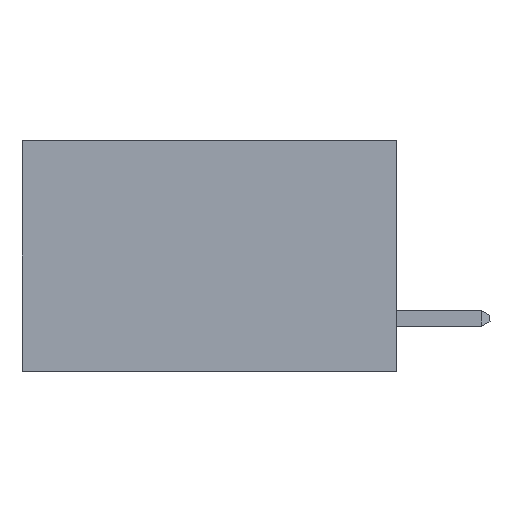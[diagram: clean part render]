
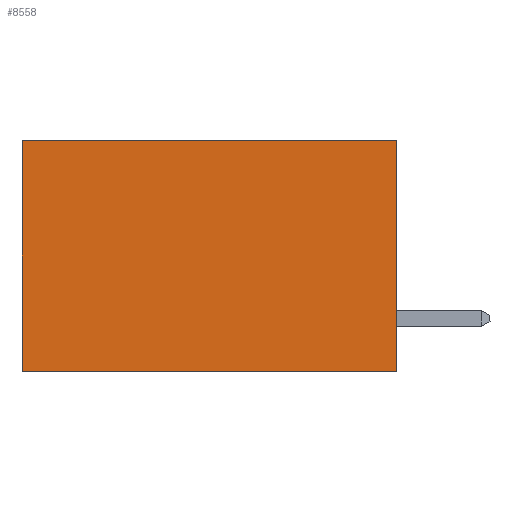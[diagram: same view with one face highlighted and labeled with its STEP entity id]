
A CAD part, left-side view. The second image highlights one B-rep face of the part: STEP entity #8558.
In plain terms, the highlighted planar face has unit normal (-1, 0, 0).
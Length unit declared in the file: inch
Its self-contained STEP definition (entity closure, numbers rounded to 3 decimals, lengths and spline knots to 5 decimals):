
#155 = LINE ( 'NONE', #3068, #6777 ) ;
#179 = DIRECTION ( 'NONE',  ( 0., 0., -1. ) ) ;
#423 = CARTESIAN_POINT ( 'NONE',  ( 0.298, 0., 0. ) ) ;
#625 = DIRECTION ( 'NONE',  ( 1., 0., 0. ) ) ;
#839 = ORIENTED_EDGE ( 'NONE', *, *, #10564, .T. ) ;
#862 = ORIENTED_EDGE ( 'NONE', *, *, #7979, .F. ) ;
#1153 = CARTESIAN_POINT ( 'NONE',  ( 0.298, 0.6, -0.37 ) ) ;
#1915 = CARTESIAN_POINT ( 'NONE',  ( 0.298, 0., 0. ) ) ;
#2089 = ORIENTED_EDGE ( 'NONE', *, *, #2822, .T. ) ;
#2137 = VERTEX_POINT ( 'NONE', #1153 ) ;
#2141 = CARTESIAN_POINT ( 'NONE',  ( 0.298, 0.6, 0. ) ) ;
#2340 = VERTEX_POINT ( 'NONE', #2141 ) ;
#2752 = CARTESIAN_POINT ( 'NONE',  ( 0.298, 0., 0. ) ) ;
#2822 = EDGE_CURVE ( 'NONE', #2340, #2137, #155, .T. ) ;
#2864 = DIRECTION ( 'NONE',  ( 0., 1., 0. ) ) ;
#3048 = VECTOR ( 'NONE', #179, 39.37008 ) ;
#3056 = DIRECTION ( 'NONE',  ( 0., 0., -1. ) ) ;
#3068 = CARTESIAN_POINT ( 'NONE',  ( 0.298, 0.6, 0. ) ) ;
#3538 = VECTOR ( 'NONE', #2864, 39.37008 ) ;
#3961 = ORIENTED_EDGE ( 'NONE', *, *, #5194, .F. ) ;
#4098 = CARTESIAN_POINT ( 'NONE',  ( 0.298, 0., -0.37 ) ) ;
#4192 = CARTESIAN_POINT ( 'NONE',  ( 0.298, 0., -0.37 ) ) ;
#4976 = VERTEX_POINT ( 'NONE', #4192 ) ;
#5194 = EDGE_CURVE ( 'NONE', #4976, #2137, #9695, .T. ) ;
#5469 = FACE_OUTER_BOUND ( 'NONE', #9498, .T. ) ;
#5515 = DIRECTION ( 'NONE',  ( 0., 1., 0. ) ) ;
#5822 = LINE ( 'NONE', #1915, #3538 ) ;
#6015 = CARTESIAN_POINT ( 'NONE',  ( 0.298, 0., 0. ) ) ;
#6777 = VECTOR ( 'NONE', #3056, 39.37008 ) ;
#6850 = DIRECTION ( 'NONE',  ( 0., 0., -1. ) ) ;
#7726 = AXIS2_PLACEMENT_3D ( 'NONE', #6015, #625, #6850 ) ;
#7857 = LINE ( 'NONE', #2752, #3048 ) ;
#7896 = VERTEX_POINT ( 'NONE', #423 ) ;
#7979 = EDGE_CURVE ( 'NONE', #7896, #4976, #7857, .T. ) ;
#8558 = ADVANCED_FACE ( 'NONE', ( #5469 ), #10990, .F. ) ;
#9173 = VECTOR ( 'NONE', #5515, 39.37008 ) ;
#9498 = EDGE_LOOP ( 'NONE', ( #2089, #3961, #862, #839 ) ) ;
#9695 = LINE ( 'NONE', #4098, #9173 ) ;
#10564 = EDGE_CURVE ( 'NONE', #7896, #2340, #5822, .T. ) ;
#10990 = PLANE ( 'NONE',  #7726 ) ;
